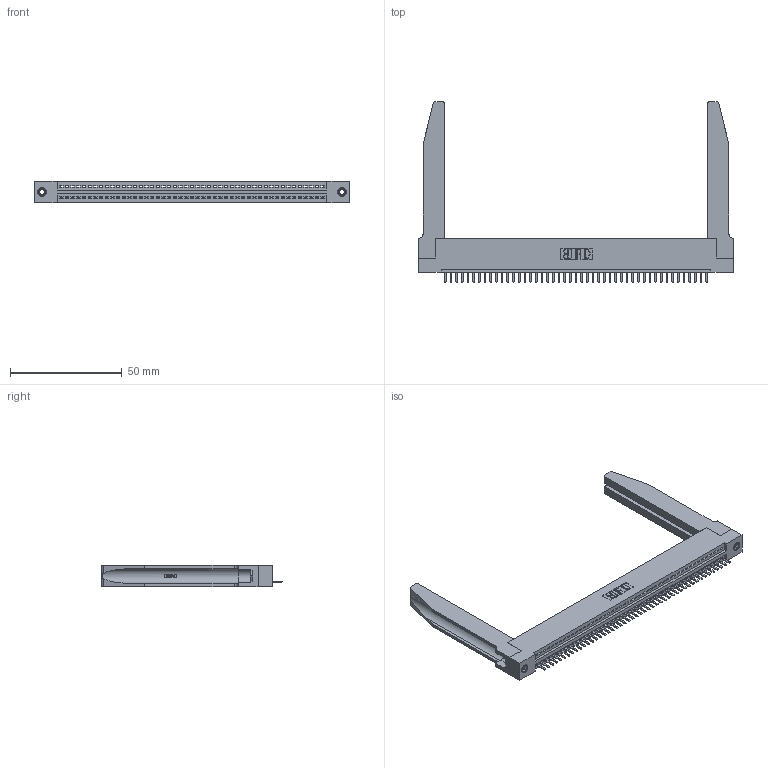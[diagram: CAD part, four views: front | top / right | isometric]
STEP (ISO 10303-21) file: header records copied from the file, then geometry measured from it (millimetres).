
FILE_DESCRIPTION (( 'STEP AP203' ), '1' );
FILE_NAME ('345-047-520-178.STEP', '2019-10-09T01:15:49', ( '' ), ( '' ), 'SwSTEP 2.0', 'SolidWorks 2016', '' );
FILE_SCHEMA (( 'CONFIG_CONTROL_DESIGN' ));
Length unit declared in the file: inch
Products named in the file (5): 345 Part_Flush Mounting Lugs - 0.156 Dia-TH; 345-250-001_345-250-001-102; 345-292-001_345-293-120; 345-047-520-178; 345-220-078_345-220-078
Assembly tree (52 placements, depth 2):
  345-047-520-178
    345 Part_Flush Mounting Lugs - 0.156 Dia-TH
    345-292-001_345-293-120  x47
    345-250-001_345-250-001-102  x2
    345-220-078_345-220-078  x2
Bounding box: 140.61 x 80.64 x 9.4 mm (x, y, z)
Volume: 21031.9 mm3; surface area: 24094.5 mm2
Topology: 52 solids, 52 shells, 3274 faces, 9597 edges, 6262 vertices
Faces by surface type: plane 2196, cylinder 1026, bspline 36, cone 12, torus 4
Entity records: 39554 total; most frequent: CARTESIAN_POINT 7760, ORIENTED_EDGE 6626, DIRECTION 5765, EDGE_CURVE 3313, LINE 2895, VECTOR 2895, VERTEX_POINT 2200, AXIS2_PLACEMENT_3D 1435
